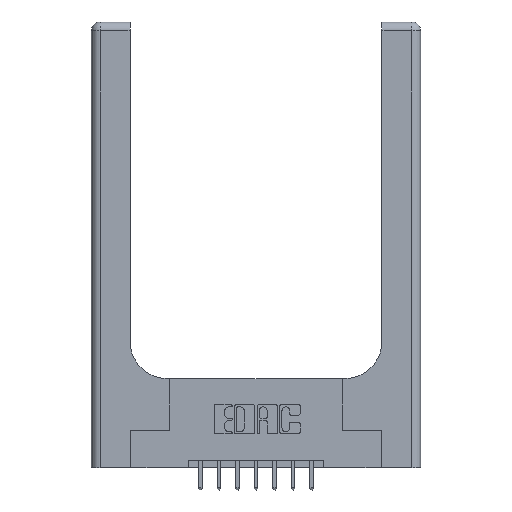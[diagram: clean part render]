
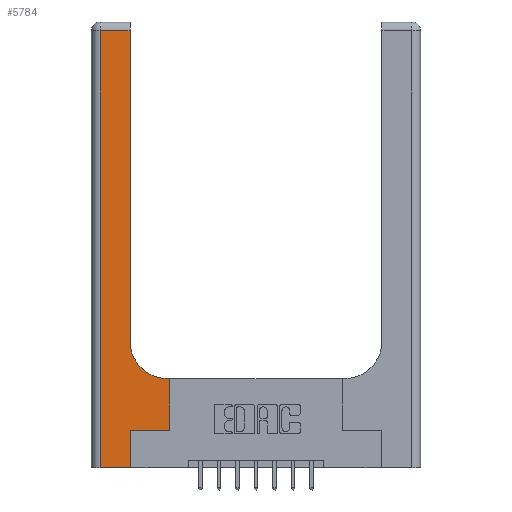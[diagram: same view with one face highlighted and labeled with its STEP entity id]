
A CAD part, top view. The second image highlights one B-rep face of the part: STEP entity #5784.
In plain terms, the highlighted planar face has unit normal (0, 0, 1).
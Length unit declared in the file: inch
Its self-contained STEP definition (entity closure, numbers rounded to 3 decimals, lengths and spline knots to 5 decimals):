
#186 = VERTEX_POINT ( 'NONE', #4080 ) ;
#483 = LINE ( 'NONE', #5389, #5657 ) ;
#670 = DIRECTION ( 'NONE',  ( 0., 1., 0. ) ) ;
#816 = ORIENTED_EDGE ( 'NONE', *, *, #8311, .T. ) ;
#833 = VECTOR ( 'NONE', #2100, 39.37008 ) ;
#938 = CARTESIAN_POINT ( 'NONE',  ( 0., 2.94, 0.37 ) ) ;
#1027 = ORIENTED_EDGE ( 'NONE', *, *, #2652, .T. ) ;
#1320 = ORIENTED_EDGE ( 'NONE', *, *, #10943, .T. ) ;
#2100 = DIRECTION ( 'NONE',  ( 0., 1., 0. ) ) ;
#2254 = VERTEX_POINT ( 'NONE', #9469 ) ;
#2282 = LINE ( 'NONE', #3505, #6811 ) ;
#2349 = VERTEX_POINT ( 'NONE', #13070 ) ;
#2590 = PLANE ( 'NONE',  #8368 ) ;
#2652 = EDGE_CURVE ( 'NONE', #2349, #2254, #14876, .T. ) ;
#2786 = ORIENTED_EDGE ( 'NONE', *, *, #11102, .T. ) ;
#3031 = CARTESIAN_POINT ( 'NONE',  ( 0., 3., 0.37 ) ) ;
#3044 = ORIENTED_EDGE ( 'NONE', *, *, #14182, .T. ) ;
#3219 = CARTESIAN_POINT ( 'NONE',  ( 0.06, 2.94, 0.37 ) ) ;
#3479 = DIRECTION ( 'NONE',  ( 1., 0., 0. ) ) ;
#3505 = CARTESIAN_POINT ( 'NONE',  ( 0.265, 0., 0.37 ) ) ;
#3801 = EDGE_CURVE ( 'NONE', #2254, #10945, #2282, .T. ) ;
#3803 = DIRECTION ( 'NONE',  ( 1., 0., 0. ) ) ;
#4080 = CARTESIAN_POINT ( 'NONE',  ( 0.51, 0.6, 0.37 ) ) ;
#4330 = EDGE_CURVE ( 'NONE', #6676, #10266, #11458, .T. ) ;
#5247 = VECTOR ( 'NONE', #670, 39.37008 ) ;
#5389 = CARTESIAN_POINT ( 'NONE',  ( 0.265, 0.25, 0.37 ) ) ;
#5533 = VERTEX_POINT ( 'NONE', #8788 ) ;
#5657 = VECTOR ( 'NONE', #9987, 39.37008 ) ;
#5784 = ADVANCED_FACE ( 'NONE', ( #12924 ), #2590, .F. ) ;
#6035 = ORIENTED_EDGE ( 'NONE', *, *, #8413, .T. ) ;
#6160 = VECTOR ( 'NONE', #11488, 39.37008 ) ;
#6361 = EDGE_CURVE ( 'NONE', #5533, #11386, #11017, .T. ) ;
#6364 = ORIENTED_EDGE ( 'NONE', *, *, #3801, .T. ) ;
#6533 = VECTOR ( 'NONE', #3479, 39.37008 ) ;
#6676 = VERTEX_POINT ( 'NONE', #11058 ) ;
#6738 = EDGE_LOOP ( 'NONE', ( #12235, #1320, #6035, #1027, #6364, #2786, #10349, #816, #3044 ) ) ;
#6811 = VECTOR ( 'NONE', #6906, 39.37008 ) ;
#6833 = LINE ( 'NONE', #938, #7656 ) ;
#6906 = DIRECTION ( 'NONE',  ( 0., 1., 0. ) ) ;
#6922 = AXIS2_PLACEMENT_3D ( 'NONE', #11865, #14124, #3803 ) ;
#7656 = VECTOR ( 'NONE', #14816, 39.37008 ) ;
#7871 = DIRECTION ( 'NONE',  ( -1., 0., 0. ) ) ;
#7880 = CIRCLE ( 'NONE', #6922, 0.25 ) ;
#7886 = CARTESIAN_POINT ( 'NONE',  ( 0.26, 0.6, 0.37 ) ) ;
#8093 = CARTESIAN_POINT ( 'NONE',  ( 0.528, 0.6, 0.37 ) ) ;
#8311 = EDGE_CURVE ( 'NONE', #10266, #186, #13679, .T. ) ;
#8368 = AXIS2_PLACEMENT_3D ( 'NONE', #3031, #13358, #7871 ) ;
#8413 = EDGE_CURVE ( 'NONE', #9235, #2349, #9398, .T. ) ;
#8788 = CARTESIAN_POINT ( 'NONE',  ( 0.26, 0.85, 0.37 ) ) ;
#8802 = VECTOR ( 'NONE', #10440, 39.37008 ) ;
#9235 = VERTEX_POINT ( 'NONE', #3219 ) ;
#9398 = LINE ( 'NONE', #12478, #6160 ) ;
#9469 = CARTESIAN_POINT ( 'NONE',  ( 0.265, 0., 0.37 ) ) ;
#9987 = DIRECTION ( 'NONE',  ( 1., 0., 0. ) ) ;
#10157 = CARTESIAN_POINT ( 'NONE',  ( 0.265, 0.25, 0.37 ) ) ;
#10266 = VERTEX_POINT ( 'NONE', #8093 ) ;
#10349 = ORIENTED_EDGE ( 'NONE', *, *, #4330, .T. ) ;
#10440 = DIRECTION ( 'NONE',  ( -1., 0., 0. ) ) ;
#10586 = CARTESIAN_POINT ( 'NONE',  ( 0., 0., 0.37 ) ) ;
#10943 = EDGE_CURVE ( 'NONE', #11386, #9235, #6833, .T. ) ;
#10945 = VERTEX_POINT ( 'NONE', #10157 ) ;
#11017 = LINE ( 'NONE', #12362, #5247 ) ;
#11058 = CARTESIAN_POINT ( 'NONE',  ( 0.528, 0.25, 0.37 ) ) ;
#11102 = EDGE_CURVE ( 'NONE', #10945, #6676, #483, .T. ) ;
#11386 = VERTEX_POINT ( 'NONE', #13894 ) ;
#11458 = LINE ( 'NONE', #11609, #833 ) ;
#11488 = DIRECTION ( 'NONE',  ( 0., -1., 0. ) ) ;
#11609 = CARTESIAN_POINT ( 'NONE',  ( 0.528, 0.25, 0.37 ) ) ;
#11865 = CARTESIAN_POINT ( 'NONE',  ( 0.51, 0.85, 0.37 ) ) ;
#12235 = ORIENTED_EDGE ( 'NONE', *, *, #6361, .T. ) ;
#12362 = CARTESIAN_POINT ( 'NONE',  ( 0.26, 3., 0.37 ) ) ;
#12478 = CARTESIAN_POINT ( 'NONE',  ( 0.06, 3., 0.37 ) ) ;
#12924 = FACE_OUTER_BOUND ( 'NONE', #6738, .T. ) ;
#13070 = CARTESIAN_POINT ( 'NONE',  ( 0.06, 0., 0.37 ) ) ;
#13358 = DIRECTION ( 'NONE',  ( 0., 0., -1. ) ) ;
#13679 = LINE ( 'NONE', #7886, #8802 ) ;
#13894 = CARTESIAN_POINT ( 'NONE',  ( 0.26, 2.94, 0.37 ) ) ;
#14124 = DIRECTION ( 'NONE',  ( 0., 0., -1. ) ) ;
#14182 = EDGE_CURVE ( 'NONE', #186, #5533, #7880, .T. ) ;
#14816 = DIRECTION ( 'NONE',  ( -1., 0., 0. ) ) ;
#14876 = LINE ( 'NONE', #10586, #6533 ) ;
